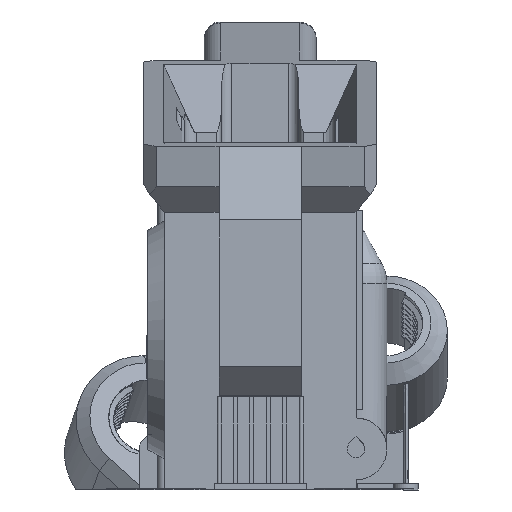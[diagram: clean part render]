
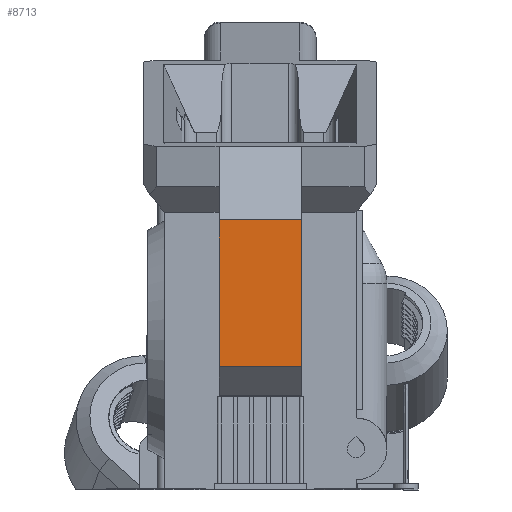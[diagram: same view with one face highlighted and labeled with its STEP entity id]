
A CAD part, left-side view. The second image highlights one B-rep face of the part: STEP entity #8713.
In plain terms, the highlighted planar face has unit normal (-1, 0, 0).
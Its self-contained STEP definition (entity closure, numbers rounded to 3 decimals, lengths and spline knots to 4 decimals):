
#8466 = EDGE_CURVE ( 'NONE', #146600, #138716, #31535, .T. ) ;
#8713 = ADVANCED_FACE ( 'NONE', ( #175623 ), #157164, .T. ) ;
#15580 = CARTESIAN_POINT ( 'NONE',  ( -4.237, 2.4558, 1.5282 ) ) ;
#22628 = LINE ( 'NONE', #55674, #89961 ) ;
#28970 = CARTESIAN_POINT ( 'NONE',  ( -4.237, 0.6526, 1.5782 ) ) ;
#31535 = LINE ( 'NONE', #38946, #177954 ) ;
#32597 = DIRECTION ( 'NONE',  ( 0., -1., 0. ) ) ;
#33223 = EDGE_CURVE ( 'NONE', #138716, #123680, #22628, .T. ) ;
#35563 = VERTEX_POINT ( 'NONE', #61117 ) ;
#38946 = CARTESIAN_POINT ( 'NONE',  ( -4.237, 0.6526, 1.5282 ) ) ;
#39351 = ORIENTED_EDGE ( 'NONE', *, *, #8466, .F. ) ;
#42483 = LINE ( 'NONE', #147710, #119048 ) ;
#43708 = EDGE_CURVE ( 'NONE', #123680, #35563, #108456, .T. ) ;
#52714 = ORIENTED_EDGE ( 'NONE', *, *, #33223, .F. ) ;
#55674 = CARTESIAN_POINT ( 'NONE',  ( -4.237, 2.4558, 1.5782 ) ) ;
#56156 = AXIS2_PLACEMENT_3D ( 'NONE', #15580, #101150, #158402 ) ;
#61117 = CARTESIAN_POINT ( 'NONE',  ( -4.237, 1.1526, 2.4712 ) ) ;
#71699 = EDGE_LOOP ( 'NONE', ( #52714, #39351, #108778, #146472 ) ) ;
#78952 = EDGE_CURVE ( 'NONE', #35563, #146600, #42483, .T. ) ;
#82329 = DIRECTION ( 'NONE',  ( 0., 0., -1. ) ) ;
#89961 = VECTOR ( 'NONE', #141294, 39.3701 ) ;
#93607 = DIRECTION ( 'NONE',  ( 0., 0., 1. ) ) ;
#101150 = DIRECTION ( 'NONE',  ( -1., 0., 0. ) ) ;
#108456 = LINE ( 'NONE', #153357, #124175 ) ;
#108778 = ORIENTED_EDGE ( 'NONE', *, *, #78952, .F. ) ;
#111678 = CARTESIAN_POINT ( 'NONE',  ( -4.237, 1.1526, 1.5782 ) ) ;
#119048 = VECTOR ( 'NONE', #32597, 39.3701 ) ;
#123680 = VERTEX_POINT ( 'NONE', #111678 ) ;
#124175 = VECTOR ( 'NONE', #93607, 39.3701 ) ;
#136561 = CARTESIAN_POINT ( 'NONE',  ( -4.237, 0.6526, 2.4712 ) ) ;
#138716 = VERTEX_POINT ( 'NONE', #28970 ) ;
#141294 = DIRECTION ( 'NONE',  ( 0., 1., 0. ) ) ;
#146472 = ORIENTED_EDGE ( 'NONE', *, *, #43708, .F. ) ;
#146600 = VERTEX_POINT ( 'NONE', #136561 ) ;
#147710 = CARTESIAN_POINT ( 'NONE',  ( -4.237, 2.4558, 2.4712 ) ) ;
#153357 = CARTESIAN_POINT ( 'NONE',  ( -4.237, 1.1526, 1.5282 ) ) ;
#157164 = PLANE ( 'NONE',  #56156 ) ;
#158402 = DIRECTION ( 'NONE',  ( 0., 0., 1. ) ) ;
#175623 = FACE_OUTER_BOUND ( 'NONE', #71699, .T. ) ;
#177954 = VECTOR ( 'NONE', #82329, 39.3701 ) ;
